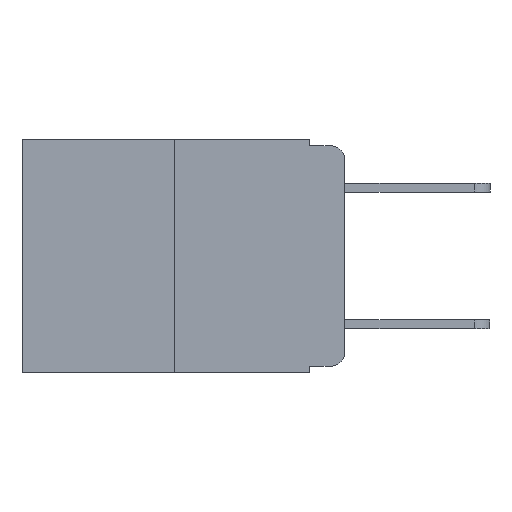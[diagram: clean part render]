
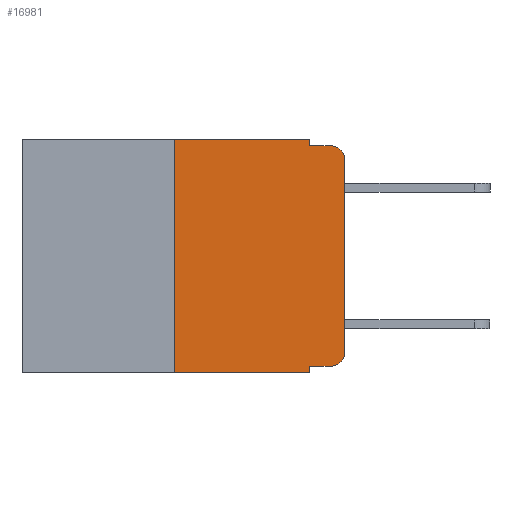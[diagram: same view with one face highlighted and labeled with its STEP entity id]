
A CAD part, left-side view. The second image highlights one B-rep face of the part: STEP entity #16981.
In plain terms, the highlighted planar face has unit normal (-1, 0, 0).
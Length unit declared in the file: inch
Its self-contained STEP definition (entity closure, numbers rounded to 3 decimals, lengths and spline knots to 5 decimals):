
#306 = AXIS2_PLACEMENT_3D ( 'NONE', #3783, #13585, #5181 ) ;
#378 = DIRECTION ( 'NONE',  ( 0., 0., -1. ) ) ;
#413 = VERTEX_POINT ( 'NONE', #12125 ) ;
#1242 = DIRECTION ( 'NONE',  ( 0., 0., 1. ) ) ;
#1480 = CARTESIAN_POINT ( 'NONE',  ( 0., 0.051, -0.333 ) ) ;
#1487 = AXIS2_PLACEMENT_3D ( 'NONE', #12094, #3699, #13509 ) ;
#1943 = ORIENTED_EDGE ( 'NONE', *, *, #9984, .F. ) ;
#2352 = VERTEX_POINT ( 'NONE', #4574 ) ;
#2458 = VECTOR ( 'NONE', #7814, 39.37008 ) ;
#2556 = EDGE_CURVE ( 'NONE', #9863, #7044, #9900, .T. ) ;
#2712 = DIRECTION ( 'NONE',  ( 0., 0., -1. ) ) ;
#2898 = DIRECTION ( 'NONE',  ( 0., -1., 0. ) ) ;
#3150 = LINE ( 'NONE', #15089, #6449 ) ;
#3234 = VERTEX_POINT ( 'NONE', #6823 ) ;
#3374 = LINE ( 'NONE', #18078, #6672 ) ;
#3699 = DIRECTION ( 'NONE',  ( -1., 0., 0. ) ) ;
#3758 = VECTOR ( 'NONE', #1242, 39.37008 ) ;
#3783 = CARTESIAN_POINT ( 'NONE',  ( 0., 0.02, -0.03 ) ) ;
#3955 = ORIENTED_EDGE ( 'NONE', *, *, #2556, .F. ) ;
#4014 = VECTOR ( 'NONE', #15648, 39.37008 ) ;
#4112 = EDGE_CURVE ( 'NONE', #413, #9863, #3150, .T. ) ;
#4447 = LINE ( 'NONE', #14235, #4014 ) ;
#4574 = CARTESIAN_POINT ( 'NONE',  ( 0., 0., -0.03 ) ) ;
#4663 = FACE_OUTER_BOUND ( 'NONE', #8028, .T. ) ;
#4981 = ORIENTED_EDGE ( 'NONE', *, *, #18079, .T. ) ;
#5181 = DIRECTION ( 'NONE',  ( 0., 0., -1. ) ) ;
#5268 = VECTOR ( 'NONE', #2898, 39.37008 ) ;
#5284 = DIRECTION ( 'NONE',  ( 0., 0., -1. ) ) ;
#5337 = EDGE_CURVE ( 'NONE', #2352, #7044, #15157, .T. ) ;
#5975 = EDGE_CURVE ( 'NONE', #12325, #11501, #16215, .T. ) ;
#6449 = VECTOR ( 'NONE', #5284, 39.37008 ) ;
#6672 = VECTOR ( 'NONE', #2712, 39.37008 ) ;
#6823 = CARTESIAN_POINT ( 'NONE',  ( 0., 0.25, -0.343 ) ) ;
#6967 = ORIENTED_EDGE ( 'NONE', *, *, #11589, .T. ) ;
#7044 = VERTEX_POINT ( 'NONE', #14815 ) ;
#7154 = CARTESIAN_POINT ( 'NONE',  ( 0., 0.051, -0.333 ) ) ;
#7469 = LINE ( 'NONE', #16611, #3758 ) ;
#7552 = ORIENTED_EDGE ( 'NONE', *, *, #13558, .F. ) ;
#7814 = DIRECTION ( 'NONE',  ( 0., -1., 0. ) ) ;
#7996 = EDGE_CURVE ( 'NONE', #8688, #12325, #16447, .T. ) ;
#8028 = EDGE_LOOP ( 'NONE', ( #6967, #9110, #3955, #12202, #1943, #7552, #4981, #12445, #10834, #15162 ) ) ;
#8553 = LINE ( 'NONE', #11457, #15558 ) ;
#8688 = VERTEX_POINT ( 'NONE', #7154 ) ;
#8725 = AXIS2_PLACEMENT_3D ( 'NONE', #14366, #8781, #378 ) ;
#8781 = DIRECTION ( 'NONE',  ( 1., 0., 0. ) ) ;
#8964 = DIRECTION ( 'NONE',  ( 0., -1., 0. ) ) ;
#9110 = ORIENTED_EDGE ( 'NONE', *, *, #5337, .T. ) ;
#9478 = CARTESIAN_POINT ( 'NONE',  ( 0., 0., -0.313 ) ) ;
#9863 = VERTEX_POINT ( 'NONE', #10060 ) ;
#9900 = LINE ( 'NONE', #14800, #2458 ) ;
#9984 = EDGE_CURVE ( 'NONE', #18155, #413, #11937, .T. ) ;
#10060 = CARTESIAN_POINT ( 'NONE',  ( 0., 0.051, -0.01 ) ) ;
#10331 = EDGE_CURVE ( 'NONE', #8688, #10486, #3374, .T. ) ;
#10486 = VERTEX_POINT ( 'NONE', #11467 ) ;
#10834 = ORIENTED_EDGE ( 'NONE', *, *, #7996, .T. ) ;
#11457 = CARTESIAN_POINT ( 'NONE',  ( 0., 0.473, -0.343 ) ) ;
#11467 = CARTESIAN_POINT ( 'NONE',  ( 0., 0.051, -0.343 ) ) ;
#11501 = VERTEX_POINT ( 'NONE', #9478 ) ;
#11589 = EDGE_CURVE ( 'NONE', #11501, #2352, #7469, .T. ) ;
#11634 = CARTESIAN_POINT ( 'NONE',  ( 0., 0.25, 0. ) ) ;
#11937 = LINE ( 'NONE', #17350, #12816 ) ;
#12094 = CARTESIAN_POINT ( 'NONE',  ( 0., 0.02, -0.313 ) ) ;
#12125 = CARTESIAN_POINT ( 'NONE',  ( 0., 0.051, 0. ) ) ;
#12202 = ORIENTED_EDGE ( 'NONE', *, *, #4112, .F. ) ;
#12325 = VERTEX_POINT ( 'NONE', #15679 ) ;
#12445 = ORIENTED_EDGE ( 'NONE', *, *, #10331, .F. ) ;
#12816 = VECTOR ( 'NONE', #8964, 39.37008 ) ;
#13509 = DIRECTION ( 'NONE',  ( 0., 0., -1. ) ) ;
#13558 = EDGE_CURVE ( 'NONE', #3234, #18155, #4447, .T. ) ;
#13585 = DIRECTION ( 'NONE',  ( -1., 0., 0. ) ) ;
#14235 = CARTESIAN_POINT ( 'NONE',  ( 0., 0.25, 0. ) ) ;
#14366 = CARTESIAN_POINT ( 'NONE',  ( 0., 0.473, 0. ) ) ;
#14800 = CARTESIAN_POINT ( 'NONE',  ( 0., 0.051, -0.01 ) ) ;
#14815 = CARTESIAN_POINT ( 'NONE',  ( 0., 0.02, -0.01 ) ) ;
#15089 = CARTESIAN_POINT ( 'NONE',  ( 0., 0.051, 0. ) ) ;
#15157 = CIRCLE ( 'NONE', #306, 0.02 ) ;
#15162 = ORIENTED_EDGE ( 'NONE', *, *, #5975, .T. ) ;
#15558 = VECTOR ( 'NONE', #17020, 39.37008 ) ;
#15648 = DIRECTION ( 'NONE',  ( 0., 0., 1. ) ) ;
#15679 = CARTESIAN_POINT ( 'NONE',  ( 0., 0.02, -0.333 ) ) ;
#16215 = CIRCLE ( 'NONE', #1487, 0.02 ) ;
#16447 = LINE ( 'NONE', #1480, #5268 ) ;
#16611 = CARTESIAN_POINT ( 'NONE',  ( 0., 0., 0. ) ) ;
#16981 = ADVANCED_FACE ( 'NONE', ( #4663 ), #17186, .F. ) ;
#17020 = DIRECTION ( 'NONE',  ( 0., -1., 0. ) ) ;
#17186 = PLANE ( 'NONE',  #8725 ) ;
#17350 = CARTESIAN_POINT ( 'NONE',  ( 0., 0.473, 0. ) ) ;
#18078 = CARTESIAN_POINT ( 'NONE',  ( 0., 0.051, 0. ) ) ;
#18079 = EDGE_CURVE ( 'NONE', #3234, #10486, #8553, .T. ) ;
#18155 = VERTEX_POINT ( 'NONE', #11634 ) ;
